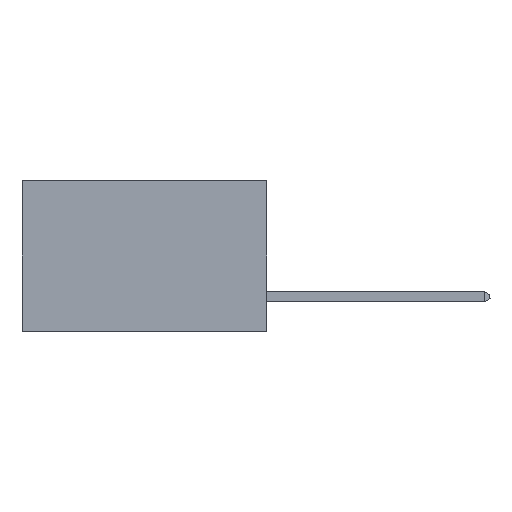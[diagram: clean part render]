
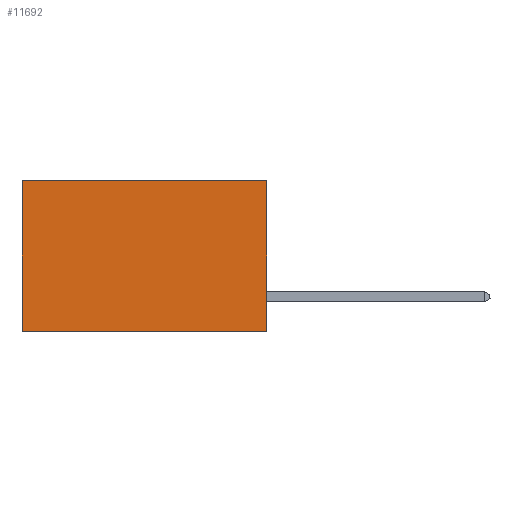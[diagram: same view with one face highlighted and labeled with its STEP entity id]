
A CAD part, left-side view. The second image highlights one B-rep face of the part: STEP entity #11692.
In plain terms, the highlighted planar face has unit normal (-1, 0, 0).
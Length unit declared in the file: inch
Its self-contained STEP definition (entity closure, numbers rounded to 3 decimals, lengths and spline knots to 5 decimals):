
#930 = EDGE_LOOP ( 'NONE', ( #22861, #1135, #32597, #30706 ) ) ;
#990 = LINE ( 'NONE', #17699, #21864 ) ;
#1129 = VERTEX_POINT ( 'NONE', #22865 ) ;
#1135 = ORIENTED_EDGE ( 'NONE', *, *, #30293, .F. ) ;
#3639 = LINE ( 'NONE', #24300, #32538 ) ;
#3872 = VECTOR ( 'NONE', #28645, 39.37008 ) ;
#4067 = DIRECTION ( 'NONE',  ( 0., 0., -1. ) ) ;
#6261 = PLANE ( 'NONE',  #8810 ) ;
#6687 = CARTESIAN_POINT ( 'NONE',  ( 0.2875, 0.6, -0.37 ) ) ;
#6799 = CARTESIAN_POINT ( 'NONE',  ( 0.2875, 0., 0. ) ) ;
#7975 = DIRECTION ( 'NONE',  ( 0., 0., -1. ) ) ;
#8409 = VERTEX_POINT ( 'NONE', #31863 ) ;
#8810 = AXIS2_PLACEMENT_3D ( 'NONE', #25345, #33414, #17294 ) ;
#9118 = VECTOR ( 'NONE', #19004, 39.37008 ) ;
#9990 = LINE ( 'NONE', #16252, #9118 ) ;
#11692 = ADVANCED_FACE ( 'NONE', ( #21464 ), #6261, .F. ) ;
#12864 = LINE ( 'NONE', #6799, #3872 ) ;
#16252 = CARTESIAN_POINT ( 'NONE',  ( 0.2875, 0., -0.37 ) ) ;
#16278 = EDGE_CURVE ( 'NONE', #29601, #23546, #3639, .T. ) ;
#17294 = DIRECTION ( 'NONE',  ( 0., 0., -1. ) ) ;
#17699 = CARTESIAN_POINT ( 'NONE',  ( 0.2875, 0., 0. ) ) ;
#19004 = DIRECTION ( 'NONE',  ( 0., 1., 0. ) ) ;
#20688 = EDGE_CURVE ( 'NONE', #1129, #8409, #990, .T. ) ;
#21464 = FACE_OUTER_BOUND ( 'NONE', #930, .T. ) ;
#21631 = EDGE_CURVE ( 'NONE', #1129, #29601, #12864, .T. ) ;
#21864 = VECTOR ( 'NONE', #4067, 39.37008 ) ;
#22861 = ORIENTED_EDGE ( 'NONE', *, *, #16278, .T. ) ;
#22865 = CARTESIAN_POINT ( 'NONE',  ( 0.2875, 0., 0. ) ) ;
#23546 = VERTEX_POINT ( 'NONE', #6687 ) ;
#23755 = CARTESIAN_POINT ( 'NONE',  ( 0.2875, 0.6, 0. ) ) ;
#24300 = CARTESIAN_POINT ( 'NONE',  ( 0.2875, 0.6, 0. ) ) ;
#25345 = CARTESIAN_POINT ( 'NONE',  ( 0.2875, 0., 0. ) ) ;
#28645 = DIRECTION ( 'NONE',  ( 0., 1., 0. ) ) ;
#29601 = VERTEX_POINT ( 'NONE', #23755 ) ;
#30293 = EDGE_CURVE ( 'NONE', #8409, #23546, #9990, .T. ) ;
#30706 = ORIENTED_EDGE ( 'NONE', *, *, #21631, .T. ) ;
#31863 = CARTESIAN_POINT ( 'NONE',  ( 0.2875, 0., -0.37 ) ) ;
#32538 = VECTOR ( 'NONE', #7975, 39.37008 ) ;
#32597 = ORIENTED_EDGE ( 'NONE', *, *, #20688, .F. ) ;
#33414 = DIRECTION ( 'NONE',  ( 1., 0., 0. ) ) ;
